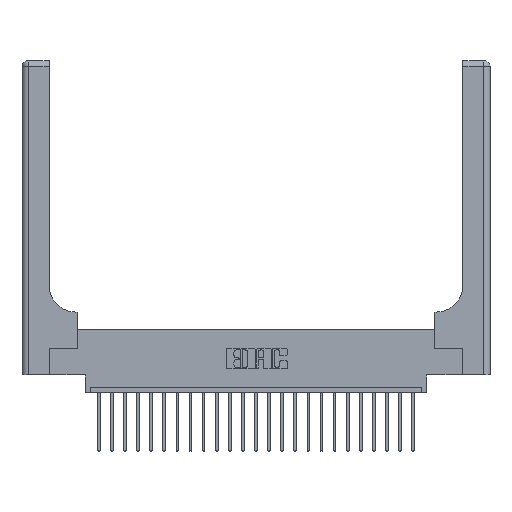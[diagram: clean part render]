
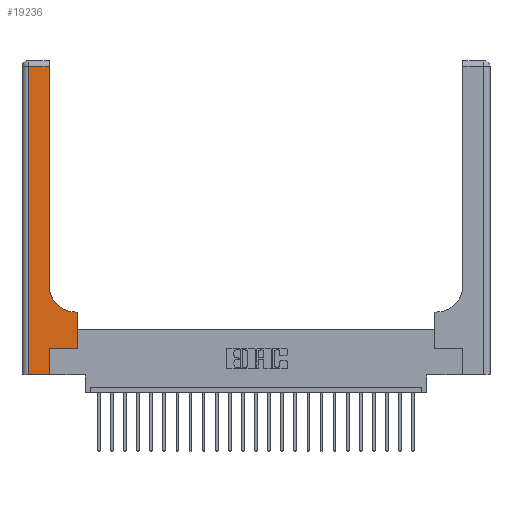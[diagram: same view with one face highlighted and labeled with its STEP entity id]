
A CAD part, top view. The second image highlights one B-rep face of the part: STEP entity #19236.
In plain terms, the highlighted planar face has unit normal (0, 0, 1).
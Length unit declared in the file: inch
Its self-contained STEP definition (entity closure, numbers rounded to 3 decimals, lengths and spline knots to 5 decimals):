
#177 = ORIENTED_EDGE ( 'NONE', *, *, #3593, .T. ) ;
#306 = ORIENTED_EDGE ( 'NONE', *, *, #2360, .T. ) ;
#364 = CARTESIAN_POINT ( 'NONE',  ( 0.528, 0.25, 0.37 ) ) ;
#1397 = DIRECTION ( 'NONE',  ( 0., 1., 0. ) ) ;
#1671 = VERTEX_POINT ( 'NONE', #2146 ) ;
#2146 = CARTESIAN_POINT ( 'NONE',  ( 0.265, 0., 0.37 ) ) ;
#2360 = EDGE_CURVE ( 'NONE', #1671, #7053, #18991, .T. ) ;
#2500 = LINE ( 'NONE', #6193, #12080 ) ;
#2712 = VECTOR ( 'NONE', #23349, 39.37008 ) ;
#2988 = ORIENTED_EDGE ( 'NONE', *, *, #17772, .T. ) ;
#3229 = VERTEX_POINT ( 'NONE', #6099 ) ;
#3593 = EDGE_CURVE ( 'NONE', #20420, #1671, #2500, .T. ) ;
#3888 = VECTOR ( 'NONE', #1397, 39.37008 ) ;
#3979 = VECTOR ( 'NONE', #13633, 39.37008 ) ;
#4585 = CARTESIAN_POINT ( 'NONE',  ( 0.265, 0., 0.37 ) ) ;
#4640 = ORIENTED_EDGE ( 'NONE', *, *, #5323, .T. ) ;
#5323 = EDGE_CURVE ( 'NONE', #20677, #19146, #15687, .T. ) ;
#5344 = DIRECTION ( 'NONE',  ( -1., 0., 0. ) ) ;
#5820 = CARTESIAN_POINT ( 'NONE',  ( 0., 2.94, 0.37 ) ) ;
#6099 = CARTESIAN_POINT ( 'NONE',  ( 0.51, 0.6, 0.37 ) ) ;
#6185 = VERTEX_POINT ( 'NONE', #15946 ) ;
#6193 = CARTESIAN_POINT ( 'NONE',  ( 0., 0., 0.37 ) ) ;
#6321 = EDGE_LOOP ( 'NONE', ( #4640, #20546, #15402, #177, #306, #22354, #8832, #2988, #21402 ) ) ;
#6539 = CARTESIAN_POINT ( 'NONE',  ( 0.528, 0.6, 0.37 ) ) ;
#6870 = LINE ( 'NONE', #12468, #18132 ) ;
#7053 = VERTEX_POINT ( 'NONE', #14567 ) ;
#7256 = AXIS2_PLACEMENT_3D ( 'NONE', #20003, #9160, #7360 ) ;
#7360 = DIRECTION ( 'NONE',  ( -1., 0., 0. ) ) ;
#8045 = VECTOR ( 'NONE', #5344, 39.37008 ) ;
#8146 = VERTEX_POINT ( 'NONE', #6539 ) ;
#8264 = EDGE_CURVE ( 'NONE', #7053, #9051, #14264, .T. ) ;
#8758 = EDGE_CURVE ( 'NONE', #9051, #8146, #13137, .T. ) ;
#8832 = ORIENTED_EDGE ( 'NONE', *, *, #8758, .T. ) ;
#9051 = VERTEX_POINT ( 'NONE', #364 ) ;
#9160 = DIRECTION ( 'NONE',  ( 0., 0., -1. ) ) ;
#9671 = DIRECTION ( 'NONE',  ( 1., 0., 0. ) ) ;
#9676 = VECTOR ( 'NONE', #12484, 39.37008 ) ;
#9864 = CIRCLE ( 'NONE', #12508, 0.25 ) ;
#11056 = EDGE_CURVE ( 'NONE', #6185, #20420, #6870, .T. ) ;
#12080 = VECTOR ( 'NONE', #15359, 39.37008 ) ;
#12376 = CARTESIAN_POINT ( 'NONE',  ( 0.26, 2.94, 0.37 ) ) ;
#12380 = CARTESIAN_POINT ( 'NONE',  ( 0.06, 0., 0.37 ) ) ;
#12468 = CARTESIAN_POINT ( 'NONE',  ( 0.06, 3., 0.37 ) ) ;
#12484 = DIRECTION ( 'NONE',  ( 1., 0., 0. ) ) ;
#12508 = AXIS2_PLACEMENT_3D ( 'NONE', #18728, #15016, #9671 ) ;
#13089 = CARTESIAN_POINT ( 'NONE',  ( 0.26, 0.85, 0.37 ) ) ;
#13137 = LINE ( 'NONE', #13255, #21112 ) ;
#13255 = CARTESIAN_POINT ( 'NONE',  ( 0.528, 0.25, 0.37 ) ) ;
#13633 = DIRECTION ( 'NONE',  ( 0., 1., 0. ) ) ;
#14013 = CARTESIAN_POINT ( 'NONE',  ( 0.26, 3., 0.37 ) ) ;
#14264 = LINE ( 'NONE', #21565, #9676 ) ;
#14392 = PLANE ( 'NONE',  #7256 ) ;
#14567 = CARTESIAN_POINT ( 'NONE',  ( 0.265, 0.25, 0.37 ) ) ;
#15016 = DIRECTION ( 'NONE',  ( 0., 0., -1. ) ) ;
#15359 = DIRECTION ( 'NONE',  ( 1., 0., 0. ) ) ;
#15402 = ORIENTED_EDGE ( 'NONE', *, *, #11056, .T. ) ;
#15687 = LINE ( 'NONE', #14013, #3888 ) ;
#15946 = CARTESIAN_POINT ( 'NONE',  ( 0.06, 2.94, 0.37 ) ) ;
#16052 = LINE ( 'NONE', #18073, #2712 ) ;
#16644 = LINE ( 'NONE', #5820, #8045 ) ;
#17601 = DIRECTION ( 'NONE',  ( 0., -1., 0. ) ) ;
#17772 = EDGE_CURVE ( 'NONE', #8146, #3229, #16052, .T. ) ;
#18073 = CARTESIAN_POINT ( 'NONE',  ( 0.26, 0.6, 0.37 ) ) ;
#18132 = VECTOR ( 'NONE', #17601, 39.37008 ) ;
#18335 = FACE_OUTER_BOUND ( 'NONE', #6321, .T. ) ;
#18728 = CARTESIAN_POINT ( 'NONE',  ( 0.51, 0.85, 0.37 ) ) ;
#18991 = LINE ( 'NONE', #4585, #3979 ) ;
#19146 = VERTEX_POINT ( 'NONE', #12376 ) ;
#19236 = ADVANCED_FACE ( 'NONE', ( #18335 ), #14392, .F. ) ;
#20003 = CARTESIAN_POINT ( 'NONE',  ( 0., 3., 0.37 ) ) ;
#20411 = DIRECTION ( 'NONE',  ( 0., 1., 0. ) ) ;
#20420 = VERTEX_POINT ( 'NONE', #12380 ) ;
#20546 = ORIENTED_EDGE ( 'NONE', *, *, #20673, .T. ) ;
#20673 = EDGE_CURVE ( 'NONE', #19146, #6185, #16644, .T. ) ;
#20677 = VERTEX_POINT ( 'NONE', #13089 ) ;
#21112 = VECTOR ( 'NONE', #20411, 39.37008 ) ;
#21402 = ORIENTED_EDGE ( 'NONE', *, *, #23412, .T. ) ;
#21565 = CARTESIAN_POINT ( 'NONE',  ( 0.265, 0.25, 0.37 ) ) ;
#22354 = ORIENTED_EDGE ( 'NONE', *, *, #8264, .T. ) ;
#23349 = DIRECTION ( 'NONE',  ( -1., 0., 0. ) ) ;
#23412 = EDGE_CURVE ( 'NONE', #3229, #20677, #9864, .T. ) ;
